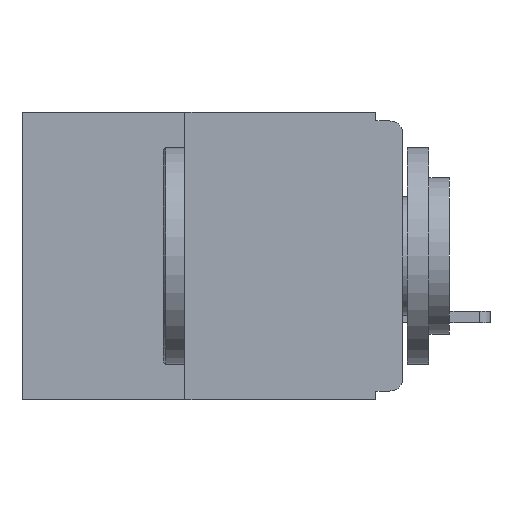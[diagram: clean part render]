
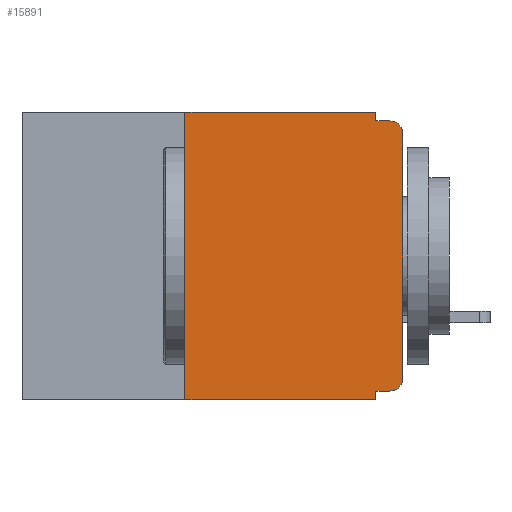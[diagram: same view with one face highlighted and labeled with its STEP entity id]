
A CAD part, left-side view. The second image highlights one B-rep face of the part: STEP entity #15891.
In plain terms, the highlighted planar face has unit normal (-1, 0, 0).
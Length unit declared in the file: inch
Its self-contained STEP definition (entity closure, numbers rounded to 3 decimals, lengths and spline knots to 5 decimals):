
#83 = CARTESIAN_POINT ( 'NONE',  ( 0., 0.031, -0.33 ) ) ;
#363 = DIRECTION ( 'NONE',  ( 0., 0., -1. ) ) ;
#518 = FACE_OUTER_BOUND ( 'NONE', #2125, .T. ) ;
#576 = CARTESIAN_POINT ( 'NONE',  ( 0., 0.015, -0.32 ) ) ;
#676 = VECTOR ( 'NONE', #363, 39.37008 ) ;
#953 = CARTESIAN_POINT ( 'NONE',  ( 0., 0.015, -0.025 ) ) ;
#1423 = EDGE_CURVE ( 'NONE', #5267, #15194, #14778, .T. ) ;
#1944 = VECTOR ( 'NONE', #13622, 39.37008 ) ;
#1972 = LINE ( 'NONE', #10306, #1944 ) ;
#2125 = EDGE_LOOP ( 'NONE', ( #8265, #8268, #8389, #8782, #8811, #8887, #8903, #9040, #9329, #9407 ) ) ;
#2222 = EDGE_CURVE ( 'NONE', #17431, #14171, #10192, .T. ) ;
#2268 = VERTEX_POINT ( 'NONE', #576 ) ;
#2462 = LINE ( 'NONE', #83, #676 ) ;
#2709 = DIRECTION ( 'NONE',  ( 0., 0., -1. ) ) ;
#3304 = VERTEX_POINT ( 'NONE', #16210 ) ;
#3549 = DIRECTION ( 'NONE',  ( -1., 0., 0. ) ) ;
#3737 = EDGE_CURVE ( 'NONE', #14171, #3304, #1972, .T. ) ;
#4205 = CARTESIAN_POINT ( 'NONE',  ( 0., 0.25, -0.33 ) ) ;
#4310 = VECTOR ( 'NONE', #11674, 39.37008 ) ;
#4397 = EDGE_CURVE ( 'NONE', #7490, #17431, #11110, .T. ) ;
#4484 = CARTESIAN_POINT ( 'NONE',  ( 0., 0.25, 0. ) ) ;
#4496 = EDGE_CURVE ( 'NONE', #3304, #15194, #17328, .T. ) ;
#4608 = CARTESIAN_POINT ( 'NONE',  ( 0., 0., -0.305 ) ) ;
#4764 = LINE ( 'NONE', #12796, #4310 ) ;
#4982 = CARTESIAN_POINT ( 'NONE',  ( 0., 0.015, -0.01 ) ) ;
#5267 = VERTEX_POINT ( 'NONE', #11147 ) ;
#6267 = EDGE_CURVE ( 'NONE', #7490, #8929, #7466, .T. ) ;
#6301 = CARTESIAN_POINT ( 'NONE',  ( 0., 0.031, 0. ) ) ;
#6366 = VERTEX_POINT ( 'NONE', #4608 ) ;
#7185 = DIRECTION ( 'NONE',  ( 0., -1., 0. ) ) ;
#7261 = CARTESIAN_POINT ( 'NONE',  ( 0., 0.437, -0.33 ) ) ;
#7313 = VECTOR ( 'NONE', #7185, 39.37008 ) ;
#7466 = LINE ( 'NONE', #7261, #7313 ) ;
#7490 = VERTEX_POINT ( 'NONE', #4205 ) ;
#7599 = AXIS2_PLACEMENT_3D ( 'NONE', #953, #3549, #2709 ) ;
#7647 = LINE ( 'NONE', #13896, #7688 ) ;
#7688 = VECTOR ( 'NONE', #14124, 39.37008 ) ;
#8259 = CARTESIAN_POINT ( 'NONE',  ( 0., 0.031, -0.33 ) ) ;
#8265 = ORIENTED_EDGE ( 'NONE', *, *, #10483, .T. ) ;
#8268 = ORIENTED_EDGE ( 'NONE', *, *, #1423, .T. ) ;
#8389 = ORIENTED_EDGE ( 'NONE', *, *, #4496, .F. ) ;
#8642 = PLANE ( 'NONE',  #15621 ) ;
#8782 = ORIENTED_EDGE ( 'NONE', *, *, #3737, .F. ) ;
#8798 = AXIS2_PLACEMENT_3D ( 'NONE', #16188, #16074, #16022 ) ;
#8811 = ORIENTED_EDGE ( 'NONE', *, *, #2222, .F. ) ;
#8887 = ORIENTED_EDGE ( 'NONE', *, *, #4397, .F. ) ;
#8903 = ORIENTED_EDGE ( 'NONE', *, *, #6267, .T. ) ;
#8929 = VERTEX_POINT ( 'NONE', #8259 ) ;
#8991 = DIRECTION ( 'NONE',  ( 0., 0., -1. ) ) ;
#9040 = ORIENTED_EDGE ( 'NONE', *, *, #9921, .F. ) ;
#9329 = ORIENTED_EDGE ( 'NONE', *, *, #16619, .F. ) ;
#9407 = ORIENTED_EDGE ( 'NONE', *, *, #10149, .T. ) ;
#9888 = VECTOR ( 'NONE', #12963, 39.37008 ) ;
#9921 = EDGE_CURVE ( 'NONE', #15983, #8929, #2462, .T. ) ;
#9969 = CARTESIAN_POINT ( 'NONE',  ( 0., 0.031, -0.32 ) ) ;
#10149 = EDGE_CURVE ( 'NONE', #2268, #6366, #14130, .T. ) ;
#10192 = LINE ( 'NONE', #18135, #9888 ) ;
#10239 = CARTESIAN_POINT ( 'NONE',  ( 0., 0.437, 0. ) ) ;
#10306 = CARTESIAN_POINT ( 'NONE',  ( 0., 0.031, 0. ) ) ;
#10483 = EDGE_CURVE ( 'NONE', #6366, #5267, #4764, .T. ) ;
#11110 = LINE ( 'NONE', #17130, #14552 ) ;
#11147 = CARTESIAN_POINT ( 'NONE',  ( 0., 0., -0.025 ) ) ;
#11674 = DIRECTION ( 'NONE',  ( 0., 0., 1. ) ) ;
#12066 = DIRECTION ( 'NONE',  ( 1., 0., 0. ) ) ;
#12796 = CARTESIAN_POINT ( 'NONE',  ( 0., 0., 0. ) ) ;
#12963 = DIRECTION ( 'NONE',  ( 0., -1., 0. ) ) ;
#12968 = DIRECTION ( 'NONE',  ( 0., -1., 0. ) ) ;
#13046 = CARTESIAN_POINT ( 'NONE',  ( 0., 0., -0.01 ) ) ;
#13622 = DIRECTION ( 'NONE',  ( 0., 0., -1. ) ) ;
#13896 = CARTESIAN_POINT ( 'NONE',  ( 0., 0., -0.32 ) ) ;
#14124 = DIRECTION ( 'NONE',  ( 0., 1., 0. ) ) ;
#14130 = CIRCLE ( 'NONE', #8798, 0.015 ) ;
#14171 = VERTEX_POINT ( 'NONE', #6301 ) ;
#14552 = VECTOR ( 'NONE', #16852, 39.37008 ) ;
#14778 = CIRCLE ( 'NONE', #7599, 0.015 ) ;
#15194 = VERTEX_POINT ( 'NONE', #4982 ) ;
#15621 = AXIS2_PLACEMENT_3D ( 'NONE', #10239, #12066, #8991 ) ;
#15891 = ADVANCED_FACE ( 'NONE', ( #518 ), #8642, .F. ) ;
#15983 = VERTEX_POINT ( 'NONE', #9969 ) ;
#16022 = DIRECTION ( 'NONE',  ( 0., 0., -1. ) ) ;
#16074 = DIRECTION ( 'NONE',  ( -1., 0., 0. ) ) ;
#16188 = CARTESIAN_POINT ( 'NONE',  ( 0., 0.015, -0.305 ) ) ;
#16210 = CARTESIAN_POINT ( 'NONE',  ( 0., 0.031, -0.01 ) ) ;
#16619 = EDGE_CURVE ( 'NONE', #2268, #15983, #7647, .T. ) ;
#16746 = VECTOR ( 'NONE', #12968, 39.37008 ) ;
#16852 = DIRECTION ( 'NONE',  ( 0., 0., 1. ) ) ;
#17130 = CARTESIAN_POINT ( 'NONE',  ( 0., 0.25, -0.33 ) ) ;
#17328 = LINE ( 'NONE', #13046, #16746 ) ;
#17431 = VERTEX_POINT ( 'NONE', #4484 ) ;
#18135 = CARTESIAN_POINT ( 'NONE',  ( 0., 0.437, 0. ) ) ;
